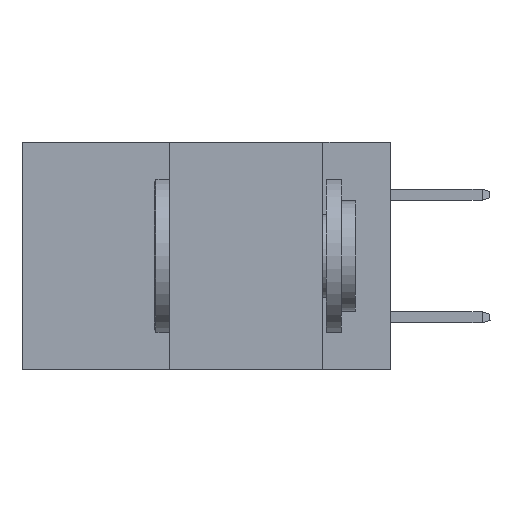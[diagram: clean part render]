
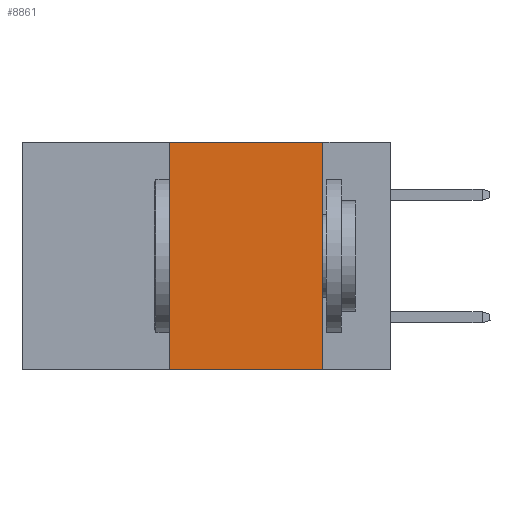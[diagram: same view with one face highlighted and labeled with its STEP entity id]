
A CAD part, left-side view. The second image highlights one B-rep face of the part: STEP entity #8861.
In plain terms, the highlighted planar face has unit normal (-1, 0, 0).
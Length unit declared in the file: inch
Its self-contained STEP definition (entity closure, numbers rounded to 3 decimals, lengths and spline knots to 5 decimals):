
#134 = LINE ( 'NONE', #2559, #11528 ) ;
#530 = CARTESIAN_POINT ( 'NONE',  ( 0., 0.11, -0.37 ) ) ;
#673 = PLANE ( 'NONE',  #13721 ) ;
#1073 = EDGE_CURVE ( 'NONE', #15356, #3874, #8385, .T. ) ;
#1745 = EDGE_CURVE ( 'NONE', #15356, #6662, #16886, .T. ) ;
#1833 = LINE ( 'NONE', #11974, #9613 ) ;
#2291 = DIRECTION ( 'NONE',  ( 1., 0., 0. ) ) ;
#2396 = ORIENTED_EDGE ( 'NONE', *, *, #3695, .F. ) ;
#2559 = CARTESIAN_POINT ( 'NONE',  ( 0., 0.6, 0. ) ) ;
#2651 = DIRECTION ( 'NONE',  ( 0., -1., 0. ) ) ;
#3695 = EDGE_CURVE ( 'NONE', #6662, #13677, #134, .T. ) ;
#3874 = VERTEX_POINT ( 'NONE', #530 ) ;
#4213 = VECTOR ( 'NONE', #18132, 39.37008 ) ;
#6100 = CARTESIAN_POINT ( 'NONE',  ( 0., 0.6, -0.37 ) ) ;
#6131 = CARTESIAN_POINT ( 'NONE',  ( 0., 0.36, -0.37 ) ) ;
#6662 = VERTEX_POINT ( 'NONE', #13792 ) ;
#7991 = DIRECTION ( 'NONE',  ( 0., 0., 1. ) ) ;
#8062 = CARTESIAN_POINT ( 'NONE',  ( 0., 0.36, 0. ) ) ;
#8385 = LINE ( 'NONE', #6100, #4213 ) ;
#8861 = ADVANCED_FACE ( 'NONE', ( #13751 ), #673, .F. ) ;
#9050 = VECTOR ( 'NONE', #7991, 39.37008 ) ;
#9613 = VECTOR ( 'NONE', #13451, 39.37008 ) ;
#10002 = CARTESIAN_POINT ( 'NONE',  ( 0., 0.6, 0. ) ) ;
#11528 = VECTOR ( 'NONE', #2651, 39.37008 ) ;
#11974 = CARTESIAN_POINT ( 'NONE',  ( 0., 0.11, 0. ) ) ;
#12210 = ORIENTED_EDGE ( 'NONE', *, *, #13237, .F. ) ;
#12697 = CARTESIAN_POINT ( 'NONE',  ( 0., 0.11, 0. ) ) ;
#12974 = DIRECTION ( 'NONE',  ( 0., 0., -1. ) ) ;
#13237 = EDGE_CURVE ( 'NONE', #13677, #3874, #1833, .T. ) ;
#13451 = DIRECTION ( 'NONE',  ( 0., 0., -1. ) ) ;
#13677 = VERTEX_POINT ( 'NONE', #12697 ) ;
#13721 = AXIS2_PLACEMENT_3D ( 'NONE', #10002, #2291, #12974 ) ;
#13751 = FACE_OUTER_BOUND ( 'NONE', #19282, .T. ) ;
#13792 = CARTESIAN_POINT ( 'NONE',  ( 0., 0.36, 0. ) ) ;
#14075 = ORIENTED_EDGE ( 'NONE', *, *, #1073, .T. ) ;
#14531 = ORIENTED_EDGE ( 'NONE', *, *, #1745, .F. ) ;
#15356 = VERTEX_POINT ( 'NONE', #6131 ) ;
#16886 = LINE ( 'NONE', #8062, #9050 ) ;
#18132 = DIRECTION ( 'NONE',  ( 0., -1., 0. ) ) ;
#19282 = EDGE_LOOP ( 'NONE', ( #12210, #2396, #14531, #14075 ) ) ;
